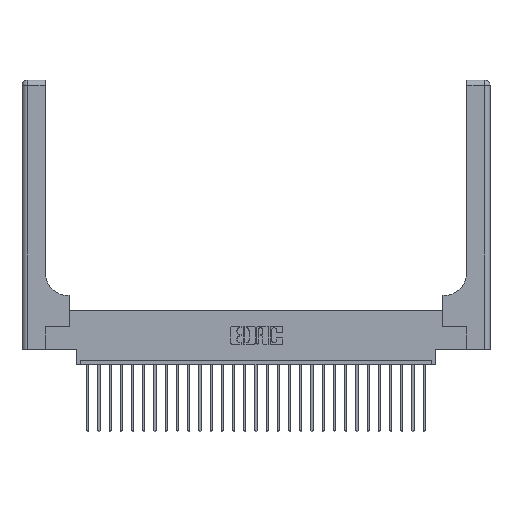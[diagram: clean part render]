
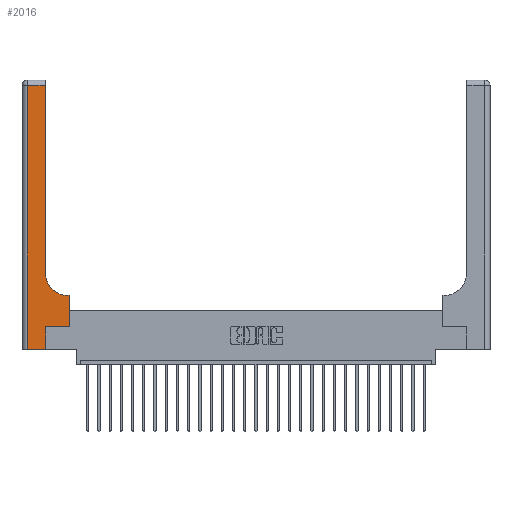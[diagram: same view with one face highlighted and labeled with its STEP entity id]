
A CAD part, top view. The second image highlights one B-rep face of the part: STEP entity #2016.
In plain terms, the highlighted planar face has unit normal (0, 0, 1).
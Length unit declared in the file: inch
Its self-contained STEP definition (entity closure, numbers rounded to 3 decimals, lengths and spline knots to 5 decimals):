
#222 = EDGE_CURVE ( 'NONE', #15632, #21739, #19973, .T. ) ;
#320 = LINE ( 'NONE', #25092, #2004 ) ;
#620 = CARTESIAN_POINT ( 'NONE',  ( 0.26, 3., 0.37 ) ) ;
#822 = CARTESIAN_POINT ( 'NONE',  ( 0.06, 2.94, 0.37 ) ) ;
#1572 = EDGE_CURVE ( 'NONE', #18077, #17604, #15721, .T. ) ;
#1644 = DIRECTION ( 'NONE',  ( 0., 1., 0. ) ) ;
#1647 = VECTOR ( 'NONE', #6231, 39.37008 ) ;
#1926 = VECTOR ( 'NONE', #12648, 39.37008 ) ;
#2004 = VECTOR ( 'NONE', #24830, 39.37008 ) ;
#2016 = ADVANCED_FACE ( 'NONE', ( #24356 ), #12025, .F. ) ;
#2296 = CARTESIAN_POINT ( 'NONE',  ( 0.51, 0.6, 0.37 ) ) ;
#2588 = ORIENTED_EDGE ( 'NONE', *, *, #222, .T. ) ;
#2619 = LINE ( 'NONE', #13046, #1926 ) ;
#3029 = CARTESIAN_POINT ( 'NONE',  ( 0.265, 0., 0.37 ) ) ;
#3491 = CARTESIAN_POINT ( 'NONE',  ( 0.528, 0.6, 0.37 ) ) ;
#3848 = VECTOR ( 'NONE', #9537, 39.37008 ) ;
#4020 = DIRECTION ( 'NONE',  ( -1., 0., 0. ) ) ;
#4338 = ORIENTED_EDGE ( 'NONE', *, *, #26128, .T. ) ;
#5077 = VERTEX_POINT ( 'NONE', #25005 ) ;
#5254 = LINE ( 'NONE', #19991, #16924 ) ;
#5972 = CARTESIAN_POINT ( 'NONE',  ( 0.528, 0.25, 0.37 ) ) ;
#6231 = DIRECTION ( 'NONE',  ( 0., 1., 0. ) ) ;
#6447 = ORIENTED_EDGE ( 'NONE', *, *, #7362, .T. ) ;
#6476 = ORIENTED_EDGE ( 'NONE', *, *, #8540, .T. ) ;
#6947 = VECTOR ( 'NONE', #4020, 39.37008 ) ;
#6969 = DIRECTION ( 'NONE',  ( 0., 0., -1. ) ) ;
#7105 = DIRECTION ( 'NONE',  ( 1., 0., 0. ) ) ;
#7362 = EDGE_CURVE ( 'NONE', #10672, #21418, #12449, .T. ) ;
#7982 = DIRECTION ( 'NONE',  ( 0., 0., -1. ) ) ;
#8355 = CIRCLE ( 'NONE', #9649, 0.25 ) ;
#8540 = EDGE_CURVE ( 'NONE', #17604, #10672, #5254, .T. ) ;
#8905 = ORIENTED_EDGE ( 'NONE', *, *, #12849, .T. ) ;
#9026 = CARTESIAN_POINT ( 'NONE',  ( 0.26, 0.85, 0.37 ) ) ;
#9027 = DIRECTION ( 'NONE',  ( 0., 1., 0. ) ) ;
#9537 = DIRECTION ( 'NONE',  ( 1., 0., 0. ) ) ;
#9649 = AXIS2_PLACEMENT_3D ( 'NONE', #22940, #6969, #7105 ) ;
#10481 = CARTESIAN_POINT ( 'NONE',  ( 0.528, 0.25, 0.37 ) ) ;
#10609 = EDGE_CURVE ( 'NONE', #21739, #14789, #8355, .T. ) ;
#10672 = VERTEX_POINT ( 'NONE', #12151 ) ;
#11052 = LINE ( 'NONE', #620, #14547 ) ;
#11890 = DIRECTION ( 'NONE',  ( -1., 0., 0. ) ) ;
#12025 = PLANE ( 'NONE',  #13093 ) ;
#12151 = CARTESIAN_POINT ( 'NONE',  ( 0.265, 0.25, 0.37 ) ) ;
#12449 = LINE ( 'NONE', #18500, #20582 ) ;
#12648 = DIRECTION ( 'NONE',  ( 0., -1., 0. ) ) ;
#12849 = EDGE_CURVE ( 'NONE', #5077, #15498, #320, .T. ) ;
#13046 = CARTESIAN_POINT ( 'NONE',  ( 0.06, 3., 0.37 ) ) ;
#13093 = AXIS2_PLACEMENT_3D ( 'NONE', #20213, #7982, #11890 ) ;
#13430 = CARTESIAN_POINT ( 'NONE',  ( 0., 0., 0.37 ) ) ;
#13886 = ORIENTED_EDGE ( 'NONE', *, *, #20915, .T. ) ;
#14547 = VECTOR ( 'NONE', #9027, 39.37008 ) ;
#14595 = EDGE_CURVE ( 'NONE', #21418, #15632, #20060, .T. ) ;
#14789 = VERTEX_POINT ( 'NONE', #9026 ) ;
#15227 = EDGE_LOOP ( 'NONE', ( #13886, #8905, #4338, #20693, #6476, #6447, #26190, #2588, #22078 ) ) ;
#15498 = VERTEX_POINT ( 'NONE', #822 ) ;
#15632 = VERTEX_POINT ( 'NONE', #3491 ) ;
#15721 = LINE ( 'NONE', #13430, #3848 ) ;
#16204 = CARTESIAN_POINT ( 'NONE',  ( 0.26, 0.6, 0.37 ) ) ;
#16924 = VECTOR ( 'NONE', #1644, 39.37008 ) ;
#17604 = VERTEX_POINT ( 'NONE', #3029 ) ;
#18077 = VERTEX_POINT ( 'NONE', #21091 ) ;
#18500 = CARTESIAN_POINT ( 'NONE',  ( 0.265, 0.25, 0.37 ) ) ;
#19973 = LINE ( 'NONE', #16204, #6947 ) ;
#19991 = CARTESIAN_POINT ( 'NONE',  ( 0.265, 0., 0.37 ) ) ;
#20060 = LINE ( 'NONE', #5972, #1647 ) ;
#20213 = CARTESIAN_POINT ( 'NONE',  ( 0., 3., 0.37 ) ) ;
#20582 = VECTOR ( 'NONE', #24271, 39.37008 ) ;
#20693 = ORIENTED_EDGE ( 'NONE', *, *, #1572, .T. ) ;
#20915 = EDGE_CURVE ( 'NONE', #14789, #5077, #11052, .T. ) ;
#21091 = CARTESIAN_POINT ( 'NONE',  ( 0.06, 0., 0.37 ) ) ;
#21418 = VERTEX_POINT ( 'NONE', #10481 ) ;
#21739 = VERTEX_POINT ( 'NONE', #2296 ) ;
#22078 = ORIENTED_EDGE ( 'NONE', *, *, #10609, .T. ) ;
#22940 = CARTESIAN_POINT ( 'NONE',  ( 0.51, 0.85, 0.37 ) ) ;
#24271 = DIRECTION ( 'NONE',  ( 1., 0., 0. ) ) ;
#24356 = FACE_OUTER_BOUND ( 'NONE', #15227, .T. ) ;
#24830 = DIRECTION ( 'NONE',  ( -1., 0., 0. ) ) ;
#25005 = CARTESIAN_POINT ( 'NONE',  ( 0.26, 2.94, 0.37 ) ) ;
#25092 = CARTESIAN_POINT ( 'NONE',  ( 0., 2.94, 0.37 ) ) ;
#26128 = EDGE_CURVE ( 'NONE', #15498, #18077, #2619, .T. ) ;
#26190 = ORIENTED_EDGE ( 'NONE', *, *, #14595, .T. ) ;
